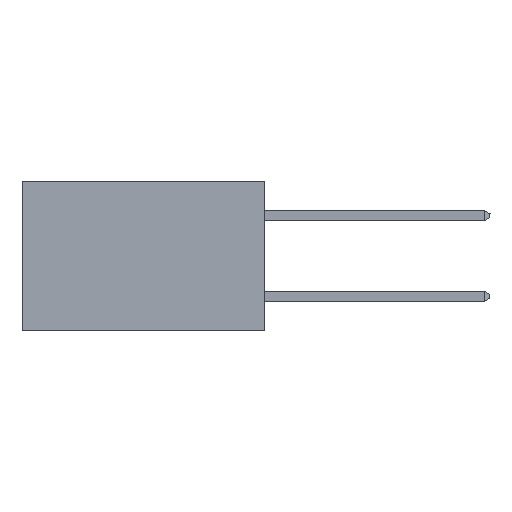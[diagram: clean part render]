
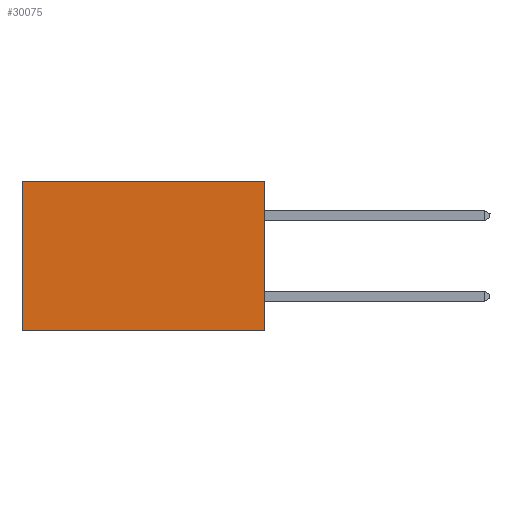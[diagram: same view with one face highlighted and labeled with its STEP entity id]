
A CAD part, left-side view. The second image highlights one B-rep face of the part: STEP entity #30075.
In plain terms, the highlighted planar face has unit normal (-1, 0, 0).
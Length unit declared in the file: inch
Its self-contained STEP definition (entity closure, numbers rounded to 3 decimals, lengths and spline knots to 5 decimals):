
#122 = DIRECTION ( 'NONE',  ( 0., 0., -1. ) ) ;
#126 = VERTEX_POINT ( 'NONE', #22859 ) ;
#198 = CARTESIAN_POINT ( 'NONE',  ( 0.298, 0., -0.37 ) ) ;
#1317 = EDGE_CURVE ( 'NONE', #29088, #28117, #32381, .T. ) ;
#2110 = VECTOR ( 'NONE', #25750, 39.37008 ) ;
#3690 = DIRECTION ( 'NONE',  ( 0., 0., -1. ) ) ;
#6650 = ORIENTED_EDGE ( 'NONE', *, *, #1317, .T. ) ;
#7623 = PLANE ( 'NONE',  #23360 ) ;
#7837 = DIRECTION ( 'NONE',  ( 0., 0., -1. ) ) ;
#11277 = CARTESIAN_POINT ( 'NONE',  ( 0.298, 0.6, 0. ) ) ;
#11820 = VERTEX_POINT ( 'NONE', #32624 ) ;
#12476 = LINE ( 'NONE', #18159, #27629 ) ;
#13340 = EDGE_CURVE ( 'NONE', #28117, #126, #32056, .T. ) ;
#13847 = FACE_OUTER_BOUND ( 'NONE', #23033, .T. ) ;
#14940 = EDGE_CURVE ( 'NONE', #11820, #126, #26430, .T. ) ;
#15723 = ORIENTED_EDGE ( 'NONE', *, *, #13340, .T. ) ;
#16523 = VECTOR ( 'NONE', #3690, 39.37008 ) ;
#18159 = CARTESIAN_POINT ( 'NONE',  ( 0.298, 0., 0. ) ) ;
#18220 = CARTESIAN_POINT ( 'NONE',  ( 0.298, 0., 0. ) ) ;
#19256 = VECTOR ( 'NONE', #31204, 39.37008 ) ;
#20950 = CARTESIAN_POINT ( 'NONE',  ( 0.298, 0., 0. ) ) ;
#22859 = CARTESIAN_POINT ( 'NONE',  ( 0.298, 0.6, -0.37 ) ) ;
#23033 = EDGE_LOOP ( 'NONE', ( #15723, #28521, #30531, #6650 ) ) ;
#23092 = CARTESIAN_POINT ( 'NONE',  ( 0.298, 0.6, 0. ) ) ;
#23208 = CARTESIAN_POINT ( 'NONE',  ( 0.298, 0., 0. ) ) ;
#23360 = AXIS2_PLACEMENT_3D ( 'NONE', #18220, #25447, #7837 ) ;
#25447 = DIRECTION ( 'NONE',  ( 1., 0., 0. ) ) ;
#25750 = DIRECTION ( 'NONE',  ( 0., 1., 0. ) ) ;
#26430 = LINE ( 'NONE', #198, #19256 ) ;
#27629 = VECTOR ( 'NONE', #122, 39.37008 ) ;
#28117 = VERTEX_POINT ( 'NONE', #23092 ) ;
#28521 = ORIENTED_EDGE ( 'NONE', *, *, #14940, .F. ) ;
#29088 = VERTEX_POINT ( 'NONE', #23208 ) ;
#30075 = ADVANCED_FACE ( 'NONE', ( #13847 ), #7623, .F. ) ;
#30531 = ORIENTED_EDGE ( 'NONE', *, *, #32230, .F. ) ;
#31204 = DIRECTION ( 'NONE',  ( 0., 1., 0. ) ) ;
#32056 = LINE ( 'NONE', #11277, #16523 ) ;
#32230 = EDGE_CURVE ( 'NONE', #29088, #11820, #12476, .T. ) ;
#32381 = LINE ( 'NONE', #20950, #2110 ) ;
#32624 = CARTESIAN_POINT ( 'NONE',  ( 0.298, 0., -0.37 ) ) ;
